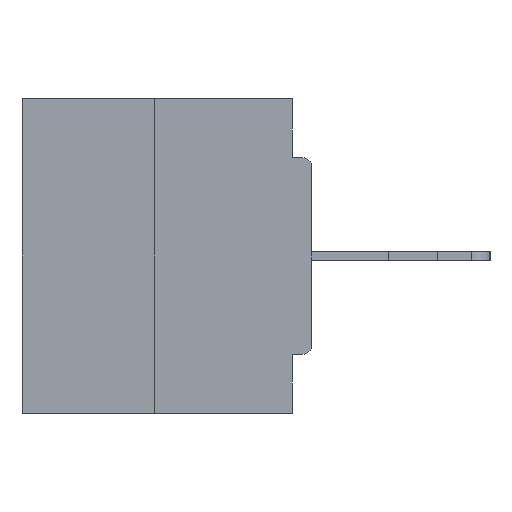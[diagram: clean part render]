
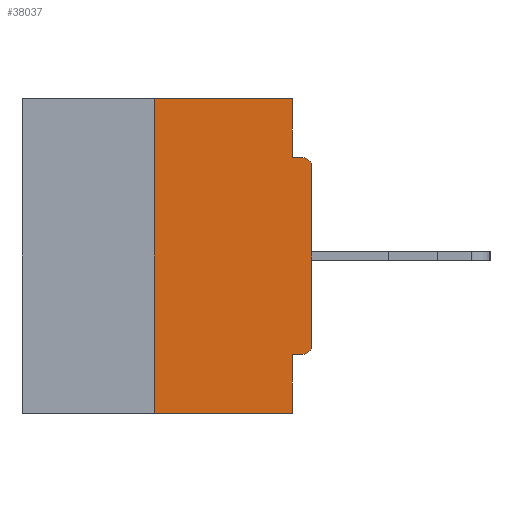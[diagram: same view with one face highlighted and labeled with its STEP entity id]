
A CAD part, left-side view. The second image highlights one B-rep face of the part: STEP entity #38037.
In plain terms, the highlighted planar face has unit normal (-1, 0, 0).
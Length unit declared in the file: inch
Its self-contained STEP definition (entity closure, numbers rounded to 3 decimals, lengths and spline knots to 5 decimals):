
#344 = VERTEX_POINT ( 'NONE', #552 ) ;
#552 = CARTESIAN_POINT ( 'NONE',  ( 0., 0.031, -0.0935 ) ) ;
#1202 = EDGE_LOOP ( 'NONE', ( #34080, #16805, #37273, #38800, #19067, #28679, #26131, #2352, #13197, #26361 ) ) ;
#1667 = VERTEX_POINT ( 'NONE', #13606 ) ;
#2157 = VECTOR ( 'NONE', #36946, 39.37008 ) ;
#2352 = ORIENTED_EDGE ( 'NONE', *, *, #26515, .T. ) ;
#2965 = CARTESIAN_POINT ( 'NONE',  ( 0., 0.031, -0.4065 ) ) ;
#3758 = CARTESIAN_POINT ( 'NONE',  ( 0., 0.015, -0.1085 ) ) ;
#4006 = DIRECTION ( 'NONE',  ( 0., 0., -1. ) ) ;
#4441 = CARTESIAN_POINT ( 'NONE',  ( 0., 0., -0.3915 ) ) ;
#4594 = CARTESIAN_POINT ( 'NONE',  ( 0., 0.015, -0.4065 ) ) ;
#5774 = LINE ( 'NONE', #33523, #2157 ) ;
#6530 = VECTOR ( 'NONE', #10104, 39.37008 ) ;
#6603 = VECTOR ( 'NONE', #34766, 39.37008 ) ;
#7415 = DIRECTION ( 'NONE',  ( -1., 0., 0. ) ) ;
#7646 = LINE ( 'NONE', #16707, #35607 ) ;
#8428 = VERTEX_POINT ( 'NONE', #24848 ) ;
#8773 = LINE ( 'NONE', #36733, #17991 ) ;
#9018 = VERTEX_POINT ( 'NONE', #32830 ) ;
#9184 = DIRECTION ( 'NONE',  ( 0., 1., 0. ) ) ;
#9502 = CARTESIAN_POINT ( 'NONE',  ( 0., 0.46, 0. ) ) ;
#10104 = DIRECTION ( 'NONE',  ( 0., -1., 0. ) ) ;
#12354 = AXIS2_PLACEMENT_3D ( 'NONE', #25008, #31461, #18411 ) ;
#12741 = EDGE_CURVE ( 'NONE', #9018, #8428, #18170, .T. ) ;
#13062 = AXIS2_PLACEMENT_3D ( 'NONE', #19262, #7415, #4006 ) ;
#13197 = ORIENTED_EDGE ( 'NONE', *, *, #17539, .F. ) ;
#13606 = CARTESIAN_POINT ( 'NONE',  ( 0., 0.031, -0.5 ) ) ;
#13968 = VERTEX_POINT ( 'NONE', #2965 ) ;
#14921 = VERTEX_POINT ( 'NONE', #4594 ) ;
#15151 = DIRECTION ( 'NONE',  ( 0., 0., 1. ) ) ;
#16063 = LINE ( 'NONE', #34981, #34089 ) ;
#16484 = CARTESIAN_POINT ( 'NONE',  ( 0., 0., 0. ) ) ;
#16707 = CARTESIAN_POINT ( 'NONE',  ( 0., 0.031, -0.5 ) ) ;
#16805 = ORIENTED_EDGE ( 'NONE', *, *, #12741, .F. ) ;
#17320 = EDGE_CURVE ( 'NONE', #38929, #28396, #22473, .T. ) ;
#17539 = EDGE_CURVE ( 'NONE', #344, #20810, #5774, .T. ) ;
#17991 = VECTOR ( 'NONE', #9184, 39.37008 ) ;
#18170 = LINE ( 'NONE', #39293, #28848 ) ;
#18411 = DIRECTION ( 'NONE',  ( 0., 0., -1. ) ) ;
#18862 = VECTOR ( 'NONE', #37581, 39.37008 ) ;
#18991 = CARTESIAN_POINT ( 'NONE',  ( 0., 0.031, 0. ) ) ;
#19067 = ORIENTED_EDGE ( 'NONE', *, *, #20448, .F. ) ;
#19205 = FACE_OUTER_BOUND ( 'NONE', #1202, .T. ) ;
#19262 = CARTESIAN_POINT ( 'NONE',  ( 0., 0.015, -0.3915 ) ) ;
#20448 = EDGE_CURVE ( 'NONE', #14921, #13968, #8773, .T. ) ;
#20810 = VERTEX_POINT ( 'NONE', #32085 ) ;
#21612 = PLANE ( 'NONE',  #12354 ) ;
#22092 = DIRECTION ( 'NONE',  ( 0., 0., -1. ) ) ;
#22359 = VERTEX_POINT ( 'NONE', #18991 ) ;
#22473 = LINE ( 'NONE', #16484, #6603 ) ;
#24848 = CARTESIAN_POINT ( 'NONE',  ( 0., 0.25, 0. ) ) ;
#25008 = CARTESIAN_POINT ( 'NONE',  ( 0., 0.46, 0. ) ) ;
#25110 = CIRCLE ( 'NONE', #28978, 0.015 ) ;
#25466 = CARTESIAN_POINT ( 'NONE',  ( 0., 0.46, -0.5 ) ) ;
#26089 = EDGE_CURVE ( 'NONE', #22359, #344, #16063, .T. ) ;
#26131 = ORIENTED_EDGE ( 'NONE', *, *, #17320, .T. ) ;
#26361 = ORIENTED_EDGE ( 'NONE', *, *, #26089, .F. ) ;
#26515 = EDGE_CURVE ( 'NONE', #28396, #20810, #25110, .T. ) ;
#27880 = DIRECTION ( 'NONE',  ( -1., 0., 0. ) ) ;
#28354 = EDGE_CURVE ( 'NONE', #9018, #1667, #34354, .T. ) ;
#28396 = VERTEX_POINT ( 'NONE', #31735 ) ;
#28486 = EDGE_CURVE ( 'NONE', #14921, #38929, #30396, .T. ) ;
#28679 = ORIENTED_EDGE ( 'NONE', *, *, #28486, .T. ) ;
#28848 = VECTOR ( 'NONE', #15151, 39.37008 ) ;
#28978 = AXIS2_PLACEMENT_3D ( 'NONE', #3758, #27880, #37124 ) ;
#29161 = DIRECTION ( 'NONE',  ( 0., 0., -1. ) ) ;
#29332 = EDGE_CURVE ( 'NONE', #13968, #1667, #7646, .T. ) ;
#30396 = CIRCLE ( 'NONE', #13062, 0.015 ) ;
#31461 = DIRECTION ( 'NONE',  ( 1., 0., 0. ) ) ;
#31735 = CARTESIAN_POINT ( 'NONE',  ( 0., 0., -0.1085 ) ) ;
#32085 = CARTESIAN_POINT ( 'NONE',  ( 0., 0.015, -0.0935 ) ) ;
#32830 = CARTESIAN_POINT ( 'NONE',  ( 0., 0.25, -0.5 ) ) ;
#33523 = CARTESIAN_POINT ( 'NONE',  ( 0., 0., -0.0935 ) ) ;
#34080 = ORIENTED_EDGE ( 'NONE', *, *, #35393, .F. ) ;
#34089 = VECTOR ( 'NONE', #22092, 39.37008 ) ;
#34354 = LINE ( 'NONE', #25466, #18862 ) ;
#34766 = DIRECTION ( 'NONE',  ( 0., 0., 1. ) ) ;
#34981 = CARTESIAN_POINT ( 'NONE',  ( 0., 0.031, 0. ) ) ;
#35393 = EDGE_CURVE ( 'NONE', #8428, #22359, #37668, .T. ) ;
#35607 = VECTOR ( 'NONE', #29161, 39.37008 ) ;
#36733 = CARTESIAN_POINT ( 'NONE',  ( 0., 0., -0.4065 ) ) ;
#36946 = DIRECTION ( 'NONE',  ( 0., -1., 0. ) ) ;
#37124 = DIRECTION ( 'NONE',  ( 0., 0., -1. ) ) ;
#37273 = ORIENTED_EDGE ( 'NONE', *, *, #28354, .T. ) ;
#37581 = DIRECTION ( 'NONE',  ( 0., -1., 0. ) ) ;
#37668 = LINE ( 'NONE', #9502, #6530 ) ;
#38037 = ADVANCED_FACE ( 'NONE', ( #19205 ), #21612, .F. ) ;
#38800 = ORIENTED_EDGE ( 'NONE', *, *, #29332, .F. ) ;
#38929 = VERTEX_POINT ( 'NONE', #4441 ) ;
#39293 = CARTESIAN_POINT ( 'NONE',  ( 0., 0.25, 0. ) ) ;
